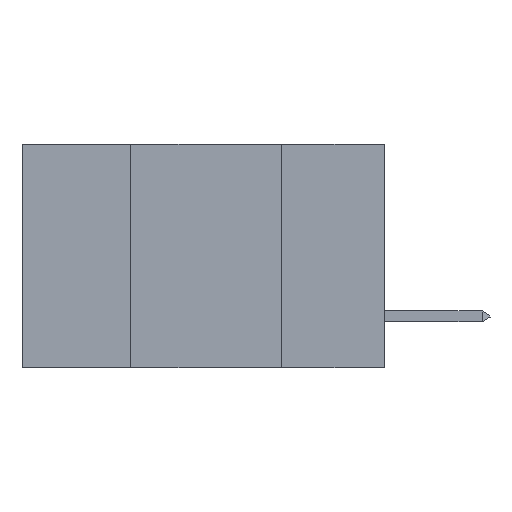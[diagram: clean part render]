
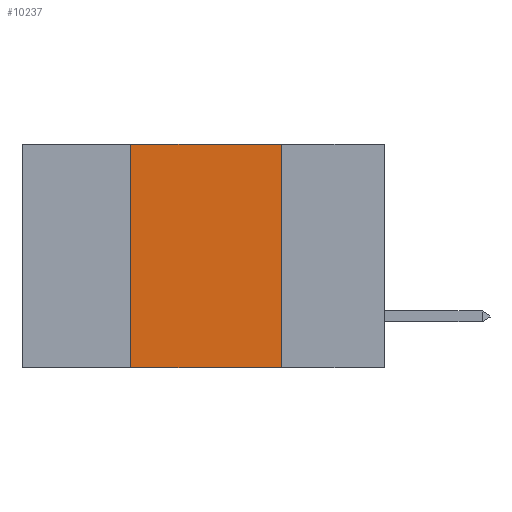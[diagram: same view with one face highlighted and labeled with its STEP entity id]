
A CAD part, left-side view. The second image highlights one B-rep face of the part: STEP entity #10237.
In plain terms, the highlighted planar face has unit normal (-1, 0, 0).
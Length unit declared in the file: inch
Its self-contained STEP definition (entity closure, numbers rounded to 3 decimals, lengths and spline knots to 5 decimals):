
#197 = VERTEX_POINT ( 'NONE', #6008 ) ;
#459 = VECTOR ( 'NONE', #7558, 39.37008 ) ;
#461 = CARTESIAN_POINT ( 'NONE',  ( 0., 0.17, 0. ) ) ;
#675 = EDGE_CURVE ( 'NONE', #6351, #6762, #9739, .T. ) ;
#795 = CARTESIAN_POINT ( 'NONE',  ( 0., 0.6, 0. ) ) ;
#945 = DIRECTION ( 'NONE',  ( 0., 0., -1. ) ) ;
#985 = ORIENTED_EDGE ( 'NONE', *, *, #6822, .F. ) ;
#992 = CARTESIAN_POINT ( 'NONE',  ( 0., 0.6, -0.37 ) ) ;
#1147 = ORIENTED_EDGE ( 'NONE', *, *, #5405, .F. ) ;
#1377 = EDGE_CURVE ( 'NONE', #6351, #197, #10621, .T. ) ;
#1737 = VERTEX_POINT ( 'NONE', #3692 ) ;
#2136 = LINE ( 'NONE', #795, #6042 ) ;
#2569 = CARTESIAN_POINT ( 'NONE',  ( 0., 0.6, 0. ) ) ;
#3373 = FACE_OUTER_BOUND ( 'NONE', #4233, .T. ) ;
#3682 = ORIENTED_EDGE ( 'NONE', *, *, #675, .T. ) ;
#3692 = CARTESIAN_POINT ( 'NONE',  ( 0., 0.17, 0. ) ) ;
#3808 = LINE ( 'NONE', #461, #5620 ) ;
#3919 = CARTESIAN_POINT ( 'NONE',  ( 0., 0.42, 0. ) ) ;
#4233 = EDGE_LOOP ( 'NONE', ( #985, #1147, #4688, #3682 ) ) ;
#4688 = ORIENTED_EDGE ( 'NONE', *, *, #1377, .F. ) ;
#5072 = DIRECTION ( 'NONE',  ( 1., 0., 0. ) ) ;
#5110 = CARTESIAN_POINT ( 'NONE',  ( 0., 0.42, -0.37 ) ) ;
#5405 = EDGE_CURVE ( 'NONE', #197, #1737, #2136, .T. ) ;
#5620 = VECTOR ( 'NONE', #9776, 39.37008 ) ;
#6008 = CARTESIAN_POINT ( 'NONE',  ( 0., 0.42, 0. ) ) ;
#6042 = VECTOR ( 'NONE', #6605, 39.37008 ) ;
#6351 = VERTEX_POINT ( 'NONE', #5110 ) ;
#6355 = AXIS2_PLACEMENT_3D ( 'NONE', #2569, #5072, #945 ) ;
#6605 = DIRECTION ( 'NONE',  ( 0., -1., 0. ) ) ;
#6762 = VERTEX_POINT ( 'NONE', #8689 ) ;
#6822 = EDGE_CURVE ( 'NONE', #1737, #6762, #3808, .T. ) ;
#7546 = PLANE ( 'NONE',  #6355 ) ;
#7558 = DIRECTION ( 'NONE',  ( 0., -1., 0. ) ) ;
#8689 = CARTESIAN_POINT ( 'NONE',  ( 0., 0.17, -0.37 ) ) ;
#8970 = DIRECTION ( 'NONE',  ( 0., 0., 1. ) ) ;
#9739 = LINE ( 'NONE', #992, #459 ) ;
#9776 = DIRECTION ( 'NONE',  ( 0., 0., -1. ) ) ;
#10237 = ADVANCED_FACE ( 'NONE', ( #3373 ), #7546, .F. ) ;
#10487 = VECTOR ( 'NONE', #8970, 39.37008 ) ;
#10621 = LINE ( 'NONE', #3919, #10487 ) ;
